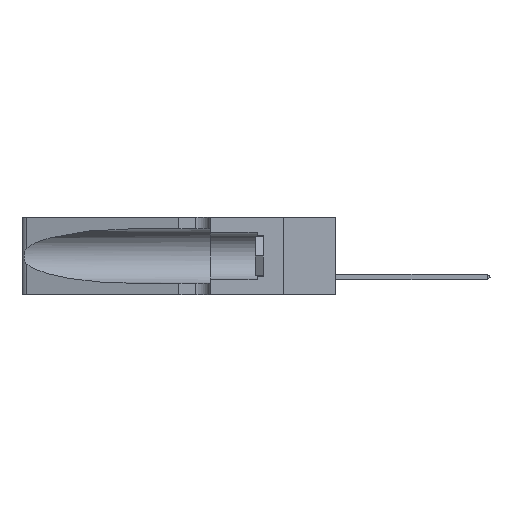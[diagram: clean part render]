
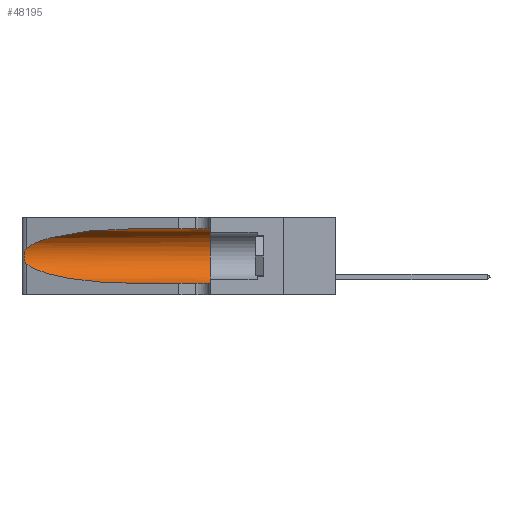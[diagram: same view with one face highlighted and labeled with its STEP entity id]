
A CAD part, left-side view. The second image highlights one B-rep face of the part: STEP entity #48195.
In plain terms, the highlighted cylindrical face has radius 3.308 mm (diameter 6.617 mm), a partial arc.
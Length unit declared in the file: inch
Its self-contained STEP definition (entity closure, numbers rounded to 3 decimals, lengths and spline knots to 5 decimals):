
#2132 = CARTESIAN_POINT ( 'NONE',  ( 0.1305, 0.72297, 0.31525 ) ) ;
#2141 = CARTESIAN_POINT ( 'NONE',  ( 0.25854, 1.2359, 0.20912 ) ) ;
#4024 = LINE ( 'NONE', #48046, #25339 ) ;
#5130 = CARTESIAN_POINT ( 'NONE',  ( 0.25856, 1.23593, 0.16098 ) ) ;
#5300 = CARTESIAN_POINT ( 'NONE',  ( 0.25639, 1.23186, 0.15144 ) ) ;
#5638 = CARTESIAN_POINT ( 'NONE',  ( 0.25787, 1.23484, 0.2124 ) ) ;
#6017 = CARTESIAN_POINT ( 'NONE',  ( 0.1305, 0.35, 0.05475 ) ) ;
#6202 = EDGE_CURVE ( 'NONE', #11987, #28258, #16588, .T. ) ;
#8270 = VECTOR ( 'NONE', #45029, 39.37008 ) ;
#9259 = CARTESIAN_POINT ( 'NONE',  ( 0.26075, 1.23896, 0.178 ) ) ;
#9437 = CARTESIAN_POINT ( 'NONE',  ( 0.25789, 1.23486, 0.15765 ) ) ;
#10394 = VERTEX_POINT ( 'NONE', #28959 ) ;
#11112 = CARTESIAN_POINT ( 'NONE',  ( 0.25487, 1.22718, 0.14631 ) ) ;
#11540 = ORIENTED_EDGE ( 'NONE', *, *, #40076, .F. ) ;
#11987 = VERTEX_POINT ( 'NONE', #34414 ) ;
#12726 = CARTESIAN_POINT ( 'NONE',  ( 0.25639, 1.23184, 0.21858 ) ) ;
#13561 = CARTESIAN_POINT ( 'NONE',  ( 0.2373, 1.15595, 0.28018 ) ) ;
#14256 = CARTESIAN_POINT ( 'NONE',  ( 0.18966, 0.96281, 0.05475 ) ) ;
#16588 = LINE ( 'NONE', #48161, #8270 ) ;
#17584 = CYLINDRICAL_SURFACE ( 'NONE', #26392, 0.13025 ) ;
#19331 = DIRECTION ( 'NONE',  ( 0., -1., 0. ) ) ;
#19356 = EDGE_CURVE ( 'NONE', #45741, #11987, #35802, .T. ) ;
#20491 = CARTESIAN_POINT ( 'NONE',  ( 0.25555, 1.22994, 0.2215 ) ) ;
#20786 = ORIENTED_EDGE ( 'NONE', *, *, #19356, .T. ) ;
#21259 = CARTESIAN_POINT ( 'NONE',  ( 0.25487, 1.22718, 0.14631 ) ) ;
#22395 = CARTESIAN_POINT ( 'NONE',  ( 0.1305, 0.72297, 0.05475 ) ) ;
#22671 = AXIS2_PLACEMENT_3D ( 'NONE', #32392, #43955, #47965 ) ;
#22785 = CARTESIAN_POINT ( 'NONE',  ( 0.1305, 0.72297, 0.31525 ) ) ;
#23653 = CIRCLE ( 'NONE', #22671, 0.13025 ) ;
#24168 = CARTESIAN_POINT ( 'NONE',  ( 0.26018, 1.23835, 0.19895 ) ) ;
#24845 = CARTESIAN_POINT ( 'NONE',  ( 0.25487, 1.22718, 0.22369 ) ) ;
#25004 = CARTESIAN_POINT ( 'NONE',  ( 0.25487, 1.22718, 0.22369 ) ) ;
#25339 = VECTOR ( 'NONE', #48564, 39.37008 ) ;
#25807 = ORIENTED_EDGE ( 'NONE', *, *, #26900, .T. ) ;
#26392 = AXIS2_PLACEMENT_3D ( 'NONE', #41858, #19331, #34006 ) ;
#26900 = EDGE_CURVE ( 'NONE', #43716, #10394, #33069, .T. ) ;
#28016 = CARTESIAN_POINT ( 'NONE',  ( 0.26075, 1.23896, 0.19203 ) ) ;
#28258 = VERTEX_POINT ( 'NONE', #6017 ) ;
#28959 = CARTESIAN_POINT ( 'NONE',  ( 0.25487, 1.22718, 0.22369 ) ) ;
#31251 = ORIENTED_EDGE ( 'NONE', *, *, #42348, .F. ) ;
#31830 = CARTESIAN_POINT ( 'NONE',  ( 0.26017, 1.23833, 0.17102 ) ) ;
#32300 = EDGE_LOOP ( 'NONE', ( #25807, #37478, #20786, #44948, #11540, #31251 ) ) ;
#32392 = CARTESIAN_POINT ( 'NONE',  ( 0.1305, 0.35, 0.185 ) ) ;
#33069 =( BOUNDED_CURVE ( )  B_SPLINE_CURVE ( 3, ( #2132, #35807, #13561, #25004 ),
 .UNSPECIFIED., .F., .F. ) 
 B_SPLINE_CURVE_WITH_KNOTS ( ( 4, 4 ),
 ( 1.5708, 2.84003 ),
 .UNSPECIFIED. ) 
 CURVE ( )  GEOMETRIC_REPRESENTATION_ITEM ( )  RATIONAL_B_SPLINE_CURVE ( ( 1., 0.87, 0.87, 1. ) ) 
 REPRESENTATION_ITEM ( '' )  );
#33740 = B_SPLINE_CURVE_WITH_KNOTS ( 'NONE', 3,
 ( #24845, #20491, #12726, #5638, #2141, #24168, #28016, #9259, #31830, #5130, #9437, #5300, #35648, #35975 ),
 .UNSPECIFIED., .F., .F.,
 ( 4, 2, 2, 2, 2, 2, 4 ),
 ( 0., 0.00027, 0.00053, 0.00107, 0.0016, 0.00187, 0.00214 ),
 .UNSPECIFIED. ) ;
#34006 = DIRECTION ( 'NONE',  ( 0., 0., -1. ) ) ;
#34414 = CARTESIAN_POINT ( 'NONE',  ( 0.1305, 0.72297, 0.05475 ) ) ;
#35349 = FACE_OUTER_BOUND ( 'NONE', #32300, .T. ) ;
#35648 = CARTESIAN_POINT ( 'NONE',  ( 0.25555, 1.22993, 0.14849 ) ) ;
#35802 =( BOUNDED_CURVE ( )  B_SPLINE_CURVE ( 3, ( #11112, #45246, #14256, #22395 ),
 .UNSPECIFIED., .F., .F. ) 
 B_SPLINE_CURVE_WITH_KNOTS ( ( 4, 4 ),
 ( 3.44316, 4.71239 ),
 .UNSPECIFIED. ) 
 CURVE ( )  GEOMETRIC_REPRESENTATION_ITEM ( )  RATIONAL_B_SPLINE_CURVE ( ( 1., 0.87, 0.87, 1. ) ) 
 REPRESENTATION_ITEM ( '' )  );
#35807 = CARTESIAN_POINT ( 'NONE',  ( 0.18966, 0.96281, 0.31525 ) ) ;
#35975 = CARTESIAN_POINT ( 'NONE',  ( 0.25487, 1.22718, 0.14631 ) ) ;
#37478 = ORIENTED_EDGE ( 'NONE', *, *, #42800, .T. ) ;
#40076 = EDGE_CURVE ( 'NONE', #47661, #28258, #23653, .T. ) ;
#41858 = CARTESIAN_POINT ( 'NONE',  ( 0.1305, 1.61858, 0.185 ) ) ;
#42348 = EDGE_CURVE ( 'NONE', #43716, #47661, #4024, .T. ) ;
#42800 = EDGE_CURVE ( 'NONE', #10394, #45741, #33740, .T. ) ;
#43716 = VERTEX_POINT ( 'NONE', #22785 ) ;
#43955 = DIRECTION ( 'NONE',  ( 0., 1., 0. ) ) ;
#44948 = ORIENTED_EDGE ( 'NONE', *, *, #6202, .T. ) ;
#45029 = DIRECTION ( 'NONE',  ( 0., -1., 0. ) ) ;
#45246 = CARTESIAN_POINT ( 'NONE',  ( 0.2373, 1.15595, 0.08982 ) ) ;
#45741 = VERTEX_POINT ( 'NONE', #21259 ) ;
#46218 = CARTESIAN_POINT ( 'NONE',  ( 0.1305, 0.35, 0.31525 ) ) ;
#47661 = VERTEX_POINT ( 'NONE', #46218 ) ;
#47965 = DIRECTION ( 'NONE',  ( 0., 0., 1. ) ) ;
#48046 = CARTESIAN_POINT ( 'NONE',  ( 0.1305, 1.61858, 0.31525 ) ) ;
#48161 = CARTESIAN_POINT ( 'NONE',  ( 0.1305, 1.61858, 0.05475 ) ) ;
#48195 = ADVANCED_FACE ( 'NONE', ( #35349 ), #17584, .F. ) ;
#48564 = DIRECTION ( 'NONE',  ( 0., -1., 0. ) ) ;
